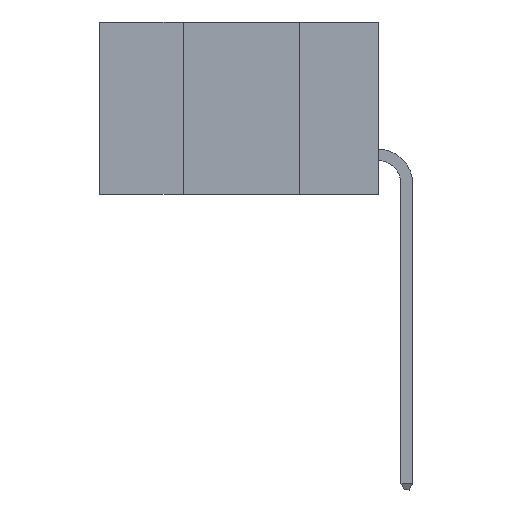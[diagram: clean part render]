
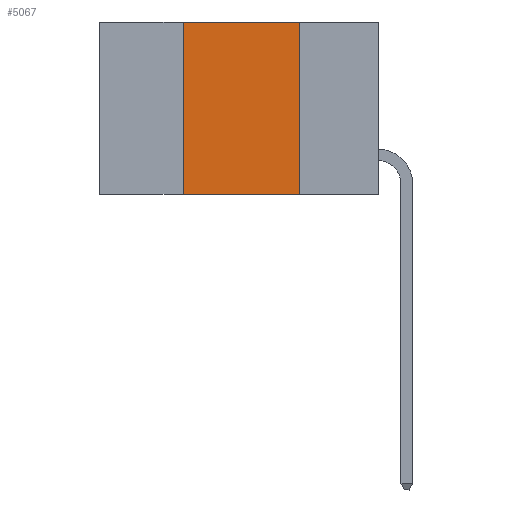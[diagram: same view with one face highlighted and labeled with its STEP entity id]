
A CAD part, left-side view. The second image highlights one B-rep face of the part: STEP entity #5067.
In plain terms, the highlighted planar face has unit normal (-1, 0, 0).
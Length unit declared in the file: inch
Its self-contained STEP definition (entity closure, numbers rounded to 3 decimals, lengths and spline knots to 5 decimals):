
#24 = FACE_OUTER_BOUND ( 'NONE', #524, .T. ) ;
#218 = DIRECTION ( 'NONE',  ( 0., 0., -1. ) ) ;
#330 = EDGE_CURVE ( 'NONE', #11458, #3082, #1868, .T. ) ;
#398 = LINE ( 'NONE', #10834, #19001 ) ;
#524 = EDGE_LOOP ( 'NONE', ( #9580, #5009, #14273, #15577 ) ) ;
#1359 = VECTOR ( 'NONE', #2533, 39.37008 ) ;
#1445 = PLANE ( 'NONE',  #7313 ) ;
#1835 = CARTESIAN_POINT ( 'NONE',  ( 0., 0.6, 0. ) ) ;
#1868 = LINE ( 'NONE', #13300, #12091 ) ;
#2533 = DIRECTION ( 'NONE',  ( 0., -1., 0. ) ) ;
#3082 = VERTEX_POINT ( 'NONE', #3506 ) ;
#3089 = DIRECTION ( 'NONE',  ( 1., 0., 0. ) ) ;
#3506 = CARTESIAN_POINT ( 'NONE',  ( 0., 0.42, 0. ) ) ;
#4316 = DIRECTION ( 'NONE',  ( 0., 0., -1. ) ) ;
#5009 = ORIENTED_EDGE ( 'NONE', *, *, #11873, .F. ) ;
#5067 = ADVANCED_FACE ( 'NONE', ( #24 ), #1445, .F. ) ;
#5072 = CARTESIAN_POINT ( 'NONE',  ( 0., 0.42, -0.37 ) ) ;
#6341 = CARTESIAN_POINT ( 'NONE',  ( 0., 0.17, 0. ) ) ;
#7020 = EDGE_CURVE ( 'NONE', #18172, #13553, #398, .T. ) ;
#7313 = AXIS2_PLACEMENT_3D ( 'NONE', #7558, #3089, #4316 ) ;
#7558 = CARTESIAN_POINT ( 'NONE',  ( 0., 0.6, 0. ) ) ;
#9580 = ORIENTED_EDGE ( 'NONE', *, *, #7020, .F. ) ;
#10101 = CARTESIAN_POINT ( 'NONE',  ( 0., 0.17, -0.37 ) ) ;
#10834 = CARTESIAN_POINT ( 'NONE',  ( 0., 0.17, 0. ) ) ;
#11195 = LINE ( 'NONE', #1835, #11663 ) ;
#11458 = VERTEX_POINT ( 'NONE', #5072 ) ;
#11663 = VECTOR ( 'NONE', #15553, 39.37008 ) ;
#11873 = EDGE_CURVE ( 'NONE', #3082, #18172, #11195, .T. ) ;
#12091 = VECTOR ( 'NONE', #14582, 39.37008 ) ;
#13300 = CARTESIAN_POINT ( 'NONE',  ( 0., 0.42, 0. ) ) ;
#13553 = VERTEX_POINT ( 'NONE', #10101 ) ;
#14273 = ORIENTED_EDGE ( 'NONE', *, *, #330, .F. ) ;
#14489 = LINE ( 'NONE', #14644, #1359 ) ;
#14582 = DIRECTION ( 'NONE',  ( 0., 0., 1. ) ) ;
#14644 = CARTESIAN_POINT ( 'NONE',  ( 0., 0.6, -0.37 ) ) ;
#14809 = EDGE_CURVE ( 'NONE', #11458, #13553, #14489, .T. ) ;
#15553 = DIRECTION ( 'NONE',  ( 0., -1., 0. ) ) ;
#15577 = ORIENTED_EDGE ( 'NONE', *, *, #14809, .T. ) ;
#18172 = VERTEX_POINT ( 'NONE', #6341 ) ;
#19001 = VECTOR ( 'NONE', #218, 39.37008 ) ;
